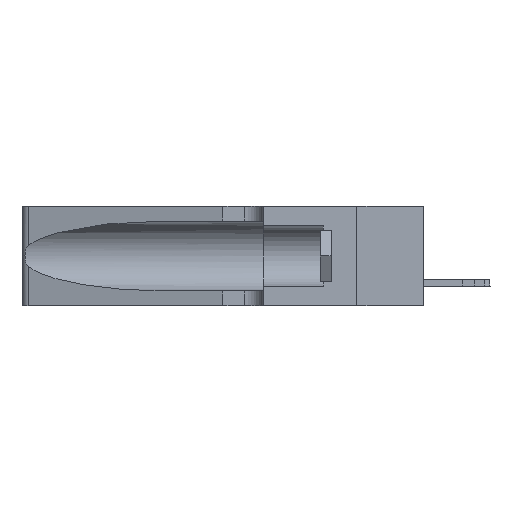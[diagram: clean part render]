
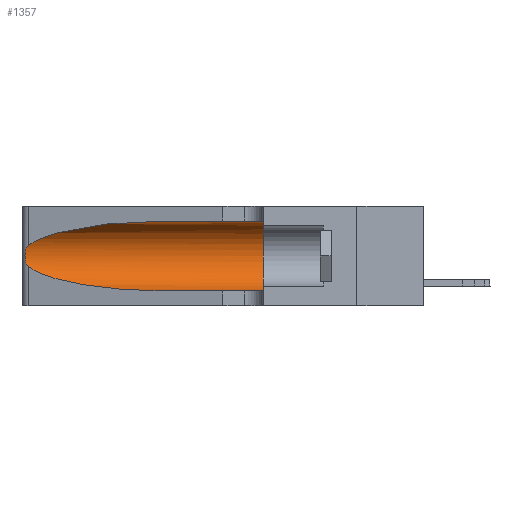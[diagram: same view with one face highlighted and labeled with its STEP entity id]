
A CAD part, left-side view. The second image highlights one B-rep face of the part: STEP entity #1357.
In plain terms, the highlighted cylindrical face has radius 3.308 mm (diameter 6.617 mm), a partial arc.
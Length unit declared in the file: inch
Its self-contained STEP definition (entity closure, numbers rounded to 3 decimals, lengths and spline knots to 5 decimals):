
#196 = B_SPLINE_CURVE_WITH_KNOTS ( 'NONE', 3,
 ( #34259, #34003, #13632, #34130, #34776, #34898, #20342, #26252, #29285, #35514, #29412, #3329, #9215, #7061 ),
 .UNSPECIFIED., .F., .F.,
 ( 4, 2, 2, 2, 2, 2, 4 ),
 ( 0., 0.00027, 0.00053, 0.00107, 0.0016, 0.00187, 0.00214 ),
 .UNSPECIFIED. ) ;
#463 = VERTEX_POINT ( 'NONE', #20377 ) ;
#1357 = ADVANCED_FACE ( 'NONE', ( #34237 ), #2133, .F. ) ;
#1664 = EDGE_CURVE ( 'NONE', #18395, #25506, #196, .T. ) ;
#1757 = CARTESIAN_POINT ( 'NONE',  ( 0.18966, 0.96281, 0.31525 ) ) ;
#1913 = CARTESIAN_POINT ( 'NONE',  ( 0.25487, 1.22718, 0.22369 ) ) ;
#2133 = CYLINDRICAL_SURFACE ( 'NONE', #30857, 0.13025 ) ;
#2850 = VERTEX_POINT ( 'NONE', #34874 ) ;
#2949 = EDGE_CURVE ( 'NONE', #463, #8728, #6120, .T. ) ;
#3329 = CARTESIAN_POINT ( 'NONE',  ( 0.25639, 1.23186, 0.15144 ) ) ;
#3698 = ORIENTED_EDGE ( 'NONE', *, *, #36998, .T. ) ;
#3830 = VECTOR ( 'NONE', #14758, 39.37008 ) ;
#5297 = CARTESIAN_POINT ( 'NONE',  ( 0.1305, 1.61858, 0.31525 ) ) ;
#5744 = CARTESIAN_POINT ( 'NONE',  ( 0.25487, 1.22718, 0.14631 ) ) ;
#5780 = CARTESIAN_POINT ( 'NONE',  ( 0.1305, 0.35, 0.05475 ) ) ;
#6120 = LINE ( 'NONE', #5297, #3830 ) ;
#6536 = CARTESIAN_POINT ( 'NONE',  ( 0.18966, 0.96281, 0.05475 ) ) ;
#7061 = CARTESIAN_POINT ( 'NONE',  ( 0.25487, 1.22718, 0.14631 ) ) ;
#8728 = VERTEX_POINT ( 'NONE', #27986 ) ;
#9215 = CARTESIAN_POINT ( 'NONE',  ( 0.25555, 1.22993, 0.14849 ) ) ;
#9879 = ORIENTED_EDGE ( 'NONE', *, *, #1664, .T. ) ;
#10534 = DIRECTION ( 'NONE',  ( 0., -1., 0. ) ) ;
#10731 = CARTESIAN_POINT ( 'NONE',  ( 0.2373, 1.15595, 0.28018 ) ) ;
#11045 =( BOUNDED_CURVE ( )  B_SPLINE_CURVE ( 3, ( #28722, #1757, #10731, #17041 ),
 .UNSPECIFIED., .F., .F. ) 
 B_SPLINE_CURVE_WITH_KNOTS ( ( 4, 4 ),
 ( 1.5708, 2.84003 ),
 .UNSPECIFIED. ) 
 CURVE ( )  GEOMETRIC_REPRESENTATION_ITEM ( )  RATIONAL_B_SPLINE_CURVE ( ( 1., 0.87, 0.87, 1. ) ) 
 REPRESENTATION_ITEM ( '' )  );
#12657 = CARTESIAN_POINT ( 'NONE',  ( 0.25487, 1.22718, 0.14631 ) ) ;
#13424 = LINE ( 'NONE', #18431, #22230 ) ;
#13632 = CARTESIAN_POINT ( 'NONE',  ( 0.25639, 1.23184, 0.21858 ) ) ;
#14758 = DIRECTION ( 'NONE',  ( 0., -1., 0. ) ) ;
#16087 = ORIENTED_EDGE ( 'NONE', *, *, #37166, .T. ) ;
#17041 = CARTESIAN_POINT ( 'NONE',  ( 0.25487, 1.22718, 0.22369 ) ) ;
#17287 = ORIENTED_EDGE ( 'NONE', *, *, #24689, .T. ) ;
#18395 = VERTEX_POINT ( 'NONE', #1913 ) ;
#18431 = CARTESIAN_POINT ( 'NONE',  ( 0.1305, 1.61858, 0.05475 ) ) ;
#19261 = DIRECTION ( 'NONE',  ( 0., 0., 1. ) ) ;
#20342 = CARTESIAN_POINT ( 'NONE',  ( 0.26075, 1.23896, 0.19203 ) ) ;
#20377 = CARTESIAN_POINT ( 'NONE',  ( 0.1305, 0.72297, 0.31525 ) ) ;
#21716 = CIRCLE ( 'NONE', #28964, 0.13025 ) ;
#21959 =( BOUNDED_CURVE ( )  B_SPLINE_CURVE ( 3, ( #12657, #24319, #6536, #29876 ),
 .UNSPECIFIED., .F., .T. ) 
 B_SPLINE_CURVE_WITH_KNOTS ( ( 4, 4 ),
 ( 3.44316, 4.71239 ),
 .UNSPECIFIED. ) 
 CURVE ( )  GEOMETRIC_REPRESENTATION_ITEM ( )  RATIONAL_B_SPLINE_CURVE ( ( 1., 0.87, 0.87, 1. ) ) 
 REPRESENTATION_ITEM ( '' )  );
#22230 = VECTOR ( 'NONE', #10534, 39.37008 ) ;
#24319 = CARTESIAN_POINT ( 'NONE',  ( 0.2373, 1.15595, 0.08982 ) ) ;
#24565 = EDGE_LOOP ( 'NONE', ( #16087, #9879, #3698, #17287, #28901, #36822 ) ) ;
#24689 = EDGE_CURVE ( 'NONE', #2850, #29750, #13424, .T. ) ;
#25506 = VERTEX_POINT ( 'NONE', #5744 ) ;
#26252 = CARTESIAN_POINT ( 'NONE',  ( 0.26075, 1.23896, 0.178 ) ) ;
#27962 = CARTESIAN_POINT ( 'NONE',  ( 0.1305, 0.35, 0.185 ) ) ;
#27986 = CARTESIAN_POINT ( 'NONE',  ( 0.1305, 0.35, 0.31525 ) ) ;
#28722 = CARTESIAN_POINT ( 'NONE',  ( 0.1305, 0.72297, 0.31525 ) ) ;
#28901 = ORIENTED_EDGE ( 'NONE', *, *, #37089, .F. ) ;
#28964 = AXIS2_PLACEMENT_3D ( 'NONE', #27962, #33679, #19261 ) ;
#29285 = CARTESIAN_POINT ( 'NONE',  ( 0.26017, 1.23833, 0.17102 ) ) ;
#29412 = CARTESIAN_POINT ( 'NONE',  ( 0.25789, 1.23486, 0.15765 ) ) ;
#29750 = VERTEX_POINT ( 'NONE', #5780 ) ;
#29876 = CARTESIAN_POINT ( 'NONE',  ( 0.1305, 0.72297, 0.05475 ) ) ;
#30857 = AXIS2_PLACEMENT_3D ( 'NONE', #31355, #34284, #30865 ) ;
#30865 = DIRECTION ( 'NONE',  ( 0., 0., -1. ) ) ;
#31355 = CARTESIAN_POINT ( 'NONE',  ( 0.1305, 1.61858, 0.185 ) ) ;
#33679 = DIRECTION ( 'NONE',  ( 0., 1., 0. ) ) ;
#34003 = CARTESIAN_POINT ( 'NONE',  ( 0.25555, 1.22994, 0.2215 ) ) ;
#34130 = CARTESIAN_POINT ( 'NONE',  ( 0.25787, 1.23484, 0.2124 ) ) ;
#34237 = FACE_OUTER_BOUND ( 'NONE', #24565, .T. ) ;
#34259 = CARTESIAN_POINT ( 'NONE',  ( 0.25487, 1.22718, 0.22369 ) ) ;
#34284 = DIRECTION ( 'NONE',  ( 0., -1., 0. ) ) ;
#34776 = CARTESIAN_POINT ( 'NONE',  ( 0.25854, 1.2359, 0.20912 ) ) ;
#34874 = CARTESIAN_POINT ( 'NONE',  ( 0.1305, 0.72297, 0.05475 ) ) ;
#34898 = CARTESIAN_POINT ( 'NONE',  ( 0.26018, 1.23835, 0.19895 ) ) ;
#35514 = CARTESIAN_POINT ( 'NONE',  ( 0.25856, 1.23593, 0.16098 ) ) ;
#36822 = ORIENTED_EDGE ( 'NONE', *, *, #2949, .F. ) ;
#36998 = EDGE_CURVE ( 'NONE', #25506, #2850, #21959, .T. ) ;
#37089 = EDGE_CURVE ( 'NONE', #8728, #29750, #21716, .T. ) ;
#37166 = EDGE_CURVE ( 'NONE', #463, #18395, #11045, .T. ) ;
